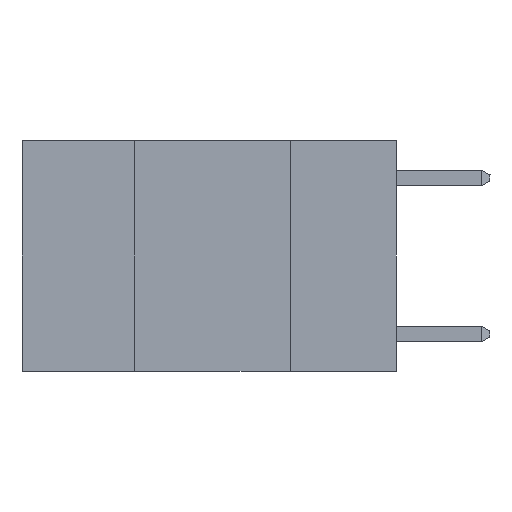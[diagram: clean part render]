
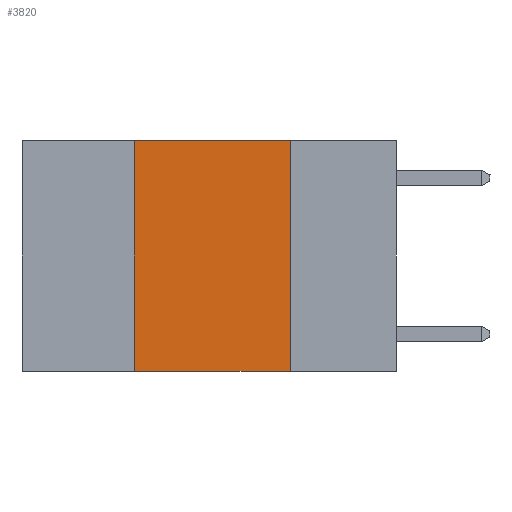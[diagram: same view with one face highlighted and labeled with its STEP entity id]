
A CAD part, left-side view. The second image highlights one B-rep face of the part: STEP entity #3820.
In plain terms, the highlighted planar face has unit normal (-1, 0, 0).
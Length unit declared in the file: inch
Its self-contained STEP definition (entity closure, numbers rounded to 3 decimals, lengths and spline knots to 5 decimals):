
#1458 = EDGE_CURVE ( 'NONE', #8423, #1714, #6703, .T. ) ;
#1714 = VERTEX_POINT ( 'NONE', #8504 ) ;
#1869 = DIRECTION ( 'NONE',  ( 0., -1., 0. ) ) ;
#1900 = CARTESIAN_POINT ( 'NONE',  ( 0., 0.17, 0. ) ) ;
#2054 = ORIENTED_EDGE ( 'NONE', *, *, #8244, .T. ) ;
#2415 = VECTOR ( 'NONE', #3503, 39.37008 ) ;
#2672 = CARTESIAN_POINT ( 'NONE',  ( 0., 0.6, -0.37 ) ) ;
#2911 = VERTEX_POINT ( 'NONE', #11152 ) ;
#3452 = VECTOR ( 'NONE', #1869, 39.37008 ) ;
#3503 = DIRECTION ( 'NONE',  ( 0., 0., 1. ) ) ;
#3549 = EDGE_LOOP ( 'NONE', ( #6205, #7837, #12210, #2054 ) ) ;
#3601 = EDGE_CURVE ( 'NONE', #6686, #2911, #8217, .T. ) ;
#3820 = ADVANCED_FACE ( 'NONE', ( #4671 ), #8460, .F. ) ;
#4118 = DIRECTION ( 'NONE',  ( 0., 0., -1. ) ) ;
#4671 = FACE_OUTER_BOUND ( 'NONE', #3549, .T. ) ;
#4790 = EDGE_CURVE ( 'NONE', #2911, #8423, #8494, .T. ) ;
#5045 = AXIS2_PLACEMENT_3D ( 'NONE', #6642, #12288, #11531 ) ;
#6205 = ORIENTED_EDGE ( 'NONE', *, *, #1458, .F. ) ;
#6225 = CARTESIAN_POINT ( 'NONE',  ( 0., 0.42, 0. ) ) ;
#6642 = CARTESIAN_POINT ( 'NONE',  ( 0., 0.6, 0. ) ) ;
#6686 = VERTEX_POINT ( 'NONE', #11748 ) ;
#6703 = LINE ( 'NONE', #1900, #10602 ) ;
#6710 = CARTESIAN_POINT ( 'NONE',  ( 0., 0.17, 0. ) ) ;
#7837 = ORIENTED_EDGE ( 'NONE', *, *, #4790, .F. ) ;
#8217 = LINE ( 'NONE', #6225, #2415 ) ;
#8244 = EDGE_CURVE ( 'NONE', #6686, #1714, #11354, .T. ) ;
#8423 = VERTEX_POINT ( 'NONE', #6710 ) ;
#8460 = PLANE ( 'NONE',  #5045 ) ;
#8494 = LINE ( 'NONE', #9323, #3452 ) ;
#8495 = VECTOR ( 'NONE', #10359, 39.37008 ) ;
#8504 = CARTESIAN_POINT ( 'NONE',  ( 0., 0.17, -0.37 ) ) ;
#9323 = CARTESIAN_POINT ( 'NONE',  ( 0., 0.6, 0. ) ) ;
#10359 = DIRECTION ( 'NONE',  ( 0., -1., 0. ) ) ;
#10602 = VECTOR ( 'NONE', #4118, 39.37008 ) ;
#11152 = CARTESIAN_POINT ( 'NONE',  ( 0., 0.42, 0. ) ) ;
#11354 = LINE ( 'NONE', #2672, #8495 ) ;
#11531 = DIRECTION ( 'NONE',  ( 0., 0., -1. ) ) ;
#11748 = CARTESIAN_POINT ( 'NONE',  ( 0., 0.42, -0.37 ) ) ;
#12210 = ORIENTED_EDGE ( 'NONE', *, *, #3601, .F. ) ;
#12288 = DIRECTION ( 'NONE',  ( 1., 0., 0. ) ) ;
